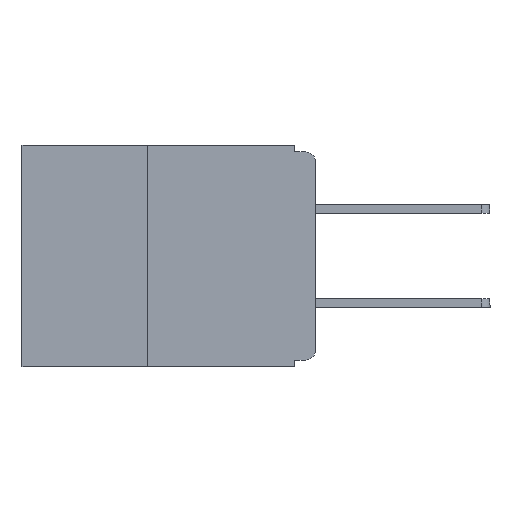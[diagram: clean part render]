
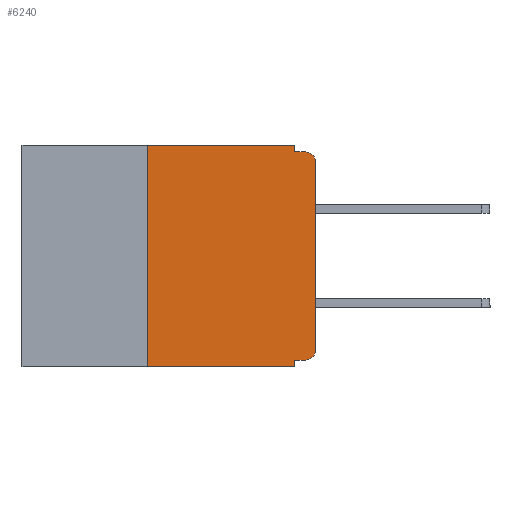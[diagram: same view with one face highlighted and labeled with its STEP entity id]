
A CAD part, left-side view. The second image highlights one B-rep face of the part: STEP entity #6240.
In plain terms, the highlighted planar face has unit normal (-1, 0, 0).
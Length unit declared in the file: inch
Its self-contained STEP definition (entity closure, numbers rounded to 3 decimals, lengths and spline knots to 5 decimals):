
#37 = DIRECTION ( 'NONE',  ( -1., 0., 0. ) ) ;
#164 = EDGE_CURVE ( 'NONE', #19000, #7441, #10180, .T. ) ;
#254 = DIRECTION ( 'NONE',  ( 0., 0., -1. ) ) ;
#1489 = ORIENTED_EDGE ( 'NONE', *, *, #1749, .T. ) ;
#1550 = CARTESIAN_POINT ( 'NONE',  ( 0., 0.015, -0.01 ) ) ;
#1617 = ORIENTED_EDGE ( 'NONE', *, *, #16400, .T. ) ;
#1749 = EDGE_CURVE ( 'NONE', #5023, #17403, #6856, .T. ) ;
#1753 = CARTESIAN_POINT ( 'NONE',  ( 0., 0., -0.01 ) ) ;
#2228 = EDGE_CURVE ( 'NONE', #11898, #19000, #11656, .T. ) ;
#2433 = AXIS2_PLACEMENT_3D ( 'NONE', #9838, #37, #11475 ) ;
#2556 = VECTOR ( 'NONE', #8834, 39.37008 ) ;
#2587 = VERTEX_POINT ( 'NONE', #18187 ) ;
#3334 = EDGE_CURVE ( 'NONE', #7950, #4726, #20676, .T. ) ;
#3410 = VERTEX_POINT ( 'NONE', #5903 ) ;
#3515 = LINE ( 'NONE', #10157, #15758 ) ;
#4203 = EDGE_CURVE ( 'NONE', #2587, #5023, #9485, .T. ) ;
#4295 = VECTOR ( 'NONE', #18036, 39.37008 ) ;
#4527 = ORIENTED_EDGE ( 'NONE', *, *, #164, .F. ) ;
#4726 = VERTEX_POINT ( 'NONE', #14378 ) ;
#5023 = VERTEX_POINT ( 'NONE', #13474 ) ;
#5264 = CARTESIAN_POINT ( 'NONE',  ( 0., 0.437, -0.33 ) ) ;
#5792 = CARTESIAN_POINT ( 'NONE',  ( 0., 0., -0.025 ) ) ;
#5903 = CARTESIAN_POINT ( 'NONE',  ( 0., 0.031, -0.33 ) ) ;
#6240 = ADVANCED_FACE ( 'NONE', ( #13443 ), #17959, .F. ) ;
#6406 = DIRECTION ( 'NONE',  ( 0., 0., -1. ) ) ;
#6634 = CARTESIAN_POINT ( 'NONE',  ( 0., 0.031, 0. ) ) ;
#6856 = LINE ( 'NONE', #14278, #2556 ) ;
#6890 = CARTESIAN_POINT ( 'NONE',  ( 0., 0.25, -0.33 ) ) ;
#6938 = DIRECTION ( 'NONE',  ( 0., 0., 1. ) ) ;
#7164 = ORIENTED_EDGE ( 'NONE', *, *, #2228, .F. ) ;
#7180 = AXIS2_PLACEMENT_3D ( 'NONE', #19521, #10052, #254 ) ;
#7325 = VECTOR ( 'NONE', #6406, 39.37008 ) ;
#7360 = CARTESIAN_POINT ( 'NONE',  ( 0., 0.031, -0.01 ) ) ;
#7441 = VERTEX_POINT ( 'NONE', #1550 ) ;
#7618 = EDGE_CURVE ( 'NONE', #7950, #3410, #12382, .T. ) ;
#7858 = CARTESIAN_POINT ( 'NONE',  ( 0., 0.031, -0.32 ) ) ;
#7950 = VERTEX_POINT ( 'NONE', #15651 ) ;
#8159 = LINE ( 'NONE', #16630, #16141 ) ;
#8298 = CARTESIAN_POINT ( 'NONE',  ( 0., 0., -0.32 ) ) ;
#8834 = DIRECTION ( 'NONE',  ( 0., 0., 1. ) ) ;
#8969 = ORIENTED_EDGE ( 'NONE', *, *, #10373, .F. ) ;
#9137 = CARTESIAN_POINT ( 'NONE',  ( 0., 0.031, 0. ) ) ;
#9279 = VERTEX_POINT ( 'NONE', #7858 ) ;
#9383 = ORIENTED_EDGE ( 'NONE', *, *, #3334, .F. ) ;
#9485 = CIRCLE ( 'NONE', #2433, 0.015 ) ;
#9704 = CARTESIAN_POINT ( 'NONE',  ( 0., 0.015, -0.025 ) ) ;
#9755 = ORIENTED_EDGE ( 'NONE', *, *, #7618, .T. ) ;
#9798 = ORIENTED_EDGE ( 'NONE', *, *, #14112, .F. ) ;
#9838 = CARTESIAN_POINT ( 'NONE',  ( 0., 0.015, -0.305 ) ) ;
#9899 = ORIENTED_EDGE ( 'NONE', *, *, #12200, .F. ) ;
#9945 = ORIENTED_EDGE ( 'NONE', *, *, #4203, .T. ) ;
#10052 = DIRECTION ( 'NONE',  ( 1., 0., 0. ) ) ;
#10157 = CARTESIAN_POINT ( 'NONE',  ( 0., 0.031, -0.33 ) ) ;
#10180 = LINE ( 'NONE', #1753, #18123 ) ;
#10373 = EDGE_CURVE ( 'NONE', #4726, #11898, #8159, .T. ) ;
#10375 = AXIS2_PLACEMENT_3D ( 'NONE', #9704, #20736, #11349 ) ;
#10887 = EDGE_LOOP ( 'NONE', ( #1489, #1617, #4527, #7164, #8969, #9383, #9755, #9798, #9899, #9945 ) ) ;
#11349 = DIRECTION ( 'NONE',  ( 0., 0., -1. ) ) ;
#11475 = DIRECTION ( 'NONE',  ( 0., 0., -1. ) ) ;
#11656 = LINE ( 'NONE', #6634, #7325 ) ;
#11790 = DIRECTION ( 'NONE',  ( 0., 0., -1. ) ) ;
#11898 = VERTEX_POINT ( 'NONE', #9137 ) ;
#12200 = EDGE_CURVE ( 'NONE', #2587, #9279, #18055, .T. ) ;
#12382 = LINE ( 'NONE', #5264, #4295 ) ;
#13443 = FACE_OUTER_BOUND ( 'NONE', #10887, .T. ) ;
#13474 = CARTESIAN_POINT ( 'NONE',  ( 0., 0., -0.305 ) ) ;
#13875 = VECTOR ( 'NONE', #17837, 39.37008 ) ;
#14051 = CIRCLE ( 'NONE', #10375, 0.015 ) ;
#14112 = EDGE_CURVE ( 'NONE', #9279, #3410, #3515, .T. ) ;
#14278 = CARTESIAN_POINT ( 'NONE',  ( 0., 0., 0. ) ) ;
#14378 = CARTESIAN_POINT ( 'NONE',  ( 0., 0.25, 0. ) ) ;
#15651 = CARTESIAN_POINT ( 'NONE',  ( 0., 0.25, -0.33 ) ) ;
#15758 = VECTOR ( 'NONE', #11790, 39.37008 ) ;
#16141 = VECTOR ( 'NONE', #19802, 39.37008 ) ;
#16400 = EDGE_CURVE ( 'NONE', #17403, #7441, #14051, .T. ) ;
#16516 = VECTOR ( 'NONE', #6938, 39.37008 ) ;
#16630 = CARTESIAN_POINT ( 'NONE',  ( 0., 0.437, 0. ) ) ;
#17403 = VERTEX_POINT ( 'NONE', #5792 ) ;
#17447 = DIRECTION ( 'NONE',  ( 0., -1., 0. ) ) ;
#17837 = DIRECTION ( 'NONE',  ( 0., 1., 0. ) ) ;
#17959 = PLANE ( 'NONE',  #7180 ) ;
#18036 = DIRECTION ( 'NONE',  ( 0., -1., 0. ) ) ;
#18055 = LINE ( 'NONE', #8298, #13875 ) ;
#18123 = VECTOR ( 'NONE', #17447, 39.37008 ) ;
#18187 = CARTESIAN_POINT ( 'NONE',  ( 0., 0.015, -0.32 ) ) ;
#19000 = VERTEX_POINT ( 'NONE', #7360 ) ;
#19521 = CARTESIAN_POINT ( 'NONE',  ( 0., 0.437, 0. ) ) ;
#19802 = DIRECTION ( 'NONE',  ( 0., -1., 0. ) ) ;
#20676 = LINE ( 'NONE', #6890, #16516 ) ;
#20736 = DIRECTION ( 'NONE',  ( -1., 0., 0. ) ) ;
